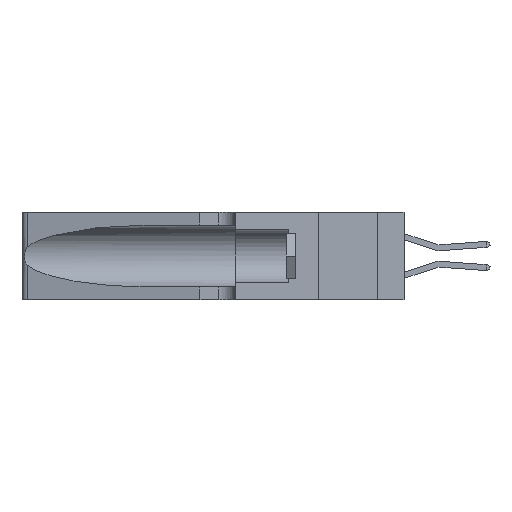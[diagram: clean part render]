
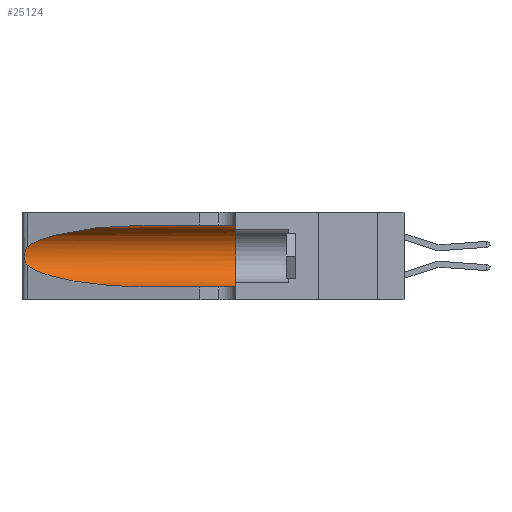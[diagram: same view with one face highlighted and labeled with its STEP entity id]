
A CAD part, left-side view. The second image highlights one B-rep face of the part: STEP entity #25124.
In plain terms, the highlighted cylindrical face has radius 3.308 mm (diameter 6.617 mm), a partial arc.
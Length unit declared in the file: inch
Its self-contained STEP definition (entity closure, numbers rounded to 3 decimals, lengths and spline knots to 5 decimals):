
#387 = VERTEX_POINT ( 'NONE', #4882 ) ;
#470 = LINE ( 'NONE', #14993, #27732 ) ;
#1335 = ORIENTED_EDGE ( 'NONE', *, *, #20385, .T. ) ;
#2355 = B_SPLINE_CURVE_WITH_KNOTS ( 'NONE', 3,
 ( #12139, #12350, #24522, #29136, #22186, #14982, #15278, #15177, #26870, #19725, #19923, #28923, #3594, #13041 ),
 .UNSPECIFIED., .F., .F.,
 ( 4, 2, 2, 2, 2, 2, 4 ),
 ( 0., 0.00027, 0.00053, 0.00107, 0.0016, 0.00187, 0.00214 ),
 .UNSPECIFIED. ) ;
#2627 = CARTESIAN_POINT ( 'NONE',  ( 0.1305, 0.35, 0.185 ) ) ;
#3594 = CARTESIAN_POINT ( 'NONE',  ( 0.25555, 1.22993, 0.14849 ) ) ;
#4491 = CARTESIAN_POINT ( 'NONE',  ( 0.1305, 0.72297, 0.31525 ) ) ;
#4882 = CARTESIAN_POINT ( 'NONE',  ( 0.25487, 1.22718, 0.22369 ) ) ;
#6069 = DIRECTION ( 'NONE',  ( 0., -1., 0. ) ) ;
#6591 = EDGE_CURVE ( 'NONE', #387, #19105, #2355, .T. ) ;
#6919 = VERTEX_POINT ( 'NONE', #4491 ) ;
#7432 = FACE_OUTER_BOUND ( 'NONE', #25870, .T. ) ;
#8242 = EDGE_CURVE ( 'NONE', #28833, #21770, #20586, .T. ) ;
#8274 = ORIENTED_EDGE ( 'NONE', *, *, #20878, .F. ) ;
#8303 = ORIENTED_EDGE ( 'NONE', *, *, #8242, .T. ) ;
#8703 = CARTESIAN_POINT ( 'NONE',  ( 0.2373, 1.15595, 0.08982 ) ) ;
#9006 = CARTESIAN_POINT ( 'NONE',  ( 0.18966, 0.96281, 0.05475 ) ) ;
#9284 = VERTEX_POINT ( 'NONE', #18604 ) ;
#10799 = ORIENTED_EDGE ( 'NONE', *, *, #24799, .T. ) ;
#11834 =( BOUNDED_CURVE ( )  B_SPLINE_CURVE ( 3, ( #20469, #8703, #9006, #25262 ),
 .UNSPECIFIED., .F., .T. ) 
 B_SPLINE_CURVE_WITH_KNOTS ( ( 4, 4 ),
 ( 3.44316, 4.71239 ),
 .UNSPECIFIED. ) 
 CURVE ( )  GEOMETRIC_REPRESENTATION_ITEM ( )  RATIONAL_B_SPLINE_CURVE ( ( 1., 0.87, 0.87, 1. ) ) 
 REPRESENTATION_ITEM ( '' )  );
#12139 = CARTESIAN_POINT ( 'NONE',  ( 0.25487, 1.22718, 0.22369 ) ) ;
#12350 = CARTESIAN_POINT ( 'NONE',  ( 0.25555, 1.22994, 0.2215 ) ) ;
#12490 = CARTESIAN_POINT ( 'NONE',  ( 0.2373, 1.15595, 0.28018 ) ) ;
#13041 = CARTESIAN_POINT ( 'NONE',  ( 0.25487, 1.22718, 0.14631 ) ) ;
#14162 = ORIENTED_EDGE ( 'NONE', *, *, #22516, .F. ) ;
#14208 = DIRECTION ( 'NONE',  ( 0., 0., 1. ) ) ;
#14433 = VECTOR ( 'NONE', #6069, 39.37008 ) ;
#14982 = CARTESIAN_POINT ( 'NONE',  ( 0.26018, 1.23835, 0.19895 ) ) ;
#14993 = CARTESIAN_POINT ( 'NONE',  ( 0.1305, 1.61858, 0.31525 ) ) ;
#15177 = CARTESIAN_POINT ( 'NONE',  ( 0.26075, 1.23896, 0.178 ) ) ;
#15278 = CARTESIAN_POINT ( 'NONE',  ( 0.26075, 1.23896, 0.19203 ) ) ;
#16207 = CIRCLE ( 'NONE', #25912, 0.13025 ) ;
#16341 = ORIENTED_EDGE ( 'NONE', *, *, #6591, .T. ) ;
#16832 = CARTESIAN_POINT ( 'NONE',  ( 0.1305, 1.61858, 0.185 ) ) ;
#17075 = CARTESIAN_POINT ( 'NONE',  ( 0.1305, 0.35, 0.05475 ) ) ;
#17567 = CARTESIAN_POINT ( 'NONE',  ( 0.1305, 0.72297, 0.05475 ) ) ;
#18144 =( BOUNDED_CURVE ( )  B_SPLINE_CURVE ( 3, ( #28464, #21412, #12490, #28672 ),
 .UNSPECIFIED., .F., .F. ) 
 B_SPLINE_CURVE_WITH_KNOTS ( ( 4, 4 ),
 ( 1.5708, 2.84003 ),
 .UNSPECIFIED. ) 
 CURVE ( )  GEOMETRIC_REPRESENTATION_ITEM ( )  RATIONAL_B_SPLINE_CURVE ( ( 1., 0.87, 0.87, 1. ) ) 
 REPRESENTATION_ITEM ( '' )  );
#18604 = CARTESIAN_POINT ( 'NONE',  ( 0.1305, 0.35, 0.31525 ) ) ;
#19105 = VERTEX_POINT ( 'NONE', #29541 ) ;
#19159 = DIRECTION ( 'NONE',  ( 0., 0., -1. ) ) ;
#19725 = CARTESIAN_POINT ( 'NONE',  ( 0.25856, 1.23593, 0.16098 ) ) ;
#19923 = CARTESIAN_POINT ( 'NONE',  ( 0.25789, 1.23486, 0.15765 ) ) ;
#20385 = EDGE_CURVE ( 'NONE', #6919, #387, #18144, .T. ) ;
#20469 = CARTESIAN_POINT ( 'NONE',  ( 0.25487, 1.22718, 0.14631 ) ) ;
#20586 = LINE ( 'NONE', #26999, #14433 ) ;
#20878 = EDGE_CURVE ( 'NONE', #9284, #21770, #16207, .T. ) ;
#21412 = CARTESIAN_POINT ( 'NONE',  ( 0.18966, 0.96281, 0.31525 ) ) ;
#21770 = VERTEX_POINT ( 'NONE', #17075 ) ;
#21897 = DIRECTION ( 'NONE',  ( 0., -1., 0. ) ) ;
#22186 = CARTESIAN_POINT ( 'NONE',  ( 0.25854, 1.2359, 0.20912 ) ) ;
#22327 = CYLINDRICAL_SURFACE ( 'NONE', #24443, 0.13025 ) ;
#22516 = EDGE_CURVE ( 'NONE', #6919, #9284, #470, .T. ) ;
#23848 = DIRECTION ( 'NONE',  ( 0., 1., 0. ) ) ;
#24443 = AXIS2_PLACEMENT_3D ( 'NONE', #16832, #25916, #19159 ) ;
#24522 = CARTESIAN_POINT ( 'NONE',  ( 0.25639, 1.23184, 0.21858 ) ) ;
#24799 = EDGE_CURVE ( 'NONE', #19105, #28833, #11834, .T. ) ;
#25124 = ADVANCED_FACE ( 'NONE', ( #7432 ), #22327, .F. ) ;
#25262 = CARTESIAN_POINT ( 'NONE',  ( 0.1305, 0.72297, 0.05475 ) ) ;
#25870 = EDGE_LOOP ( 'NONE', ( #1335, #16341, #10799, #8303, #8274, #14162 ) ) ;
#25912 = AXIS2_PLACEMENT_3D ( 'NONE', #2627, #23848, #14208 ) ;
#25916 = DIRECTION ( 'NONE',  ( 0., -1., 0. ) ) ;
#26870 = CARTESIAN_POINT ( 'NONE',  ( 0.26017, 1.23833, 0.17102 ) ) ;
#26999 = CARTESIAN_POINT ( 'NONE',  ( 0.1305, 1.61858, 0.05475 ) ) ;
#27732 = VECTOR ( 'NONE', #21897, 39.37008 ) ;
#28464 = CARTESIAN_POINT ( 'NONE',  ( 0.1305, 0.72297, 0.31525 ) ) ;
#28672 = CARTESIAN_POINT ( 'NONE',  ( 0.25487, 1.22718, 0.22369 ) ) ;
#28833 = VERTEX_POINT ( 'NONE', #17567 ) ;
#28923 = CARTESIAN_POINT ( 'NONE',  ( 0.25639, 1.23186, 0.15144 ) ) ;
#29136 = CARTESIAN_POINT ( 'NONE',  ( 0.25787, 1.23484, 0.2124 ) ) ;
#29541 = CARTESIAN_POINT ( 'NONE',  ( 0.25487, 1.22718, 0.14631 ) ) ;
